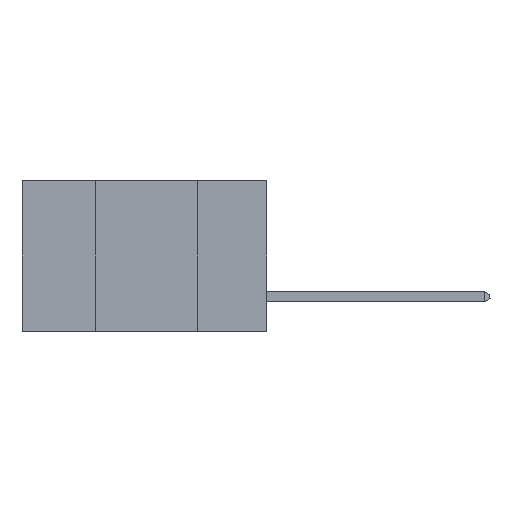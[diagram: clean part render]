
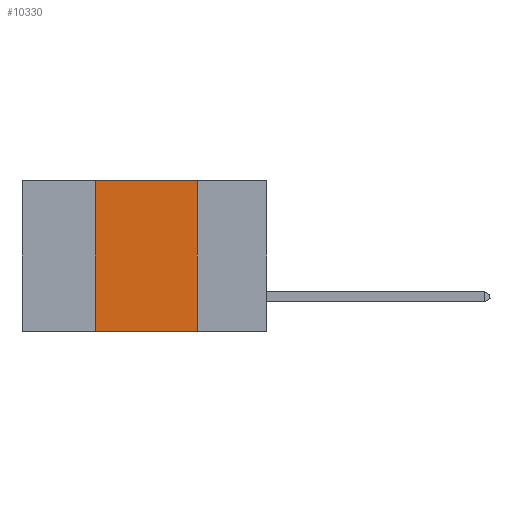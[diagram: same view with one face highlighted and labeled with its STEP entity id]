
A CAD part, left-side view. The second image highlights one B-rep face of the part: STEP entity #10330.
In plain terms, the highlighted planar face has unit normal (-1, 0, 0).
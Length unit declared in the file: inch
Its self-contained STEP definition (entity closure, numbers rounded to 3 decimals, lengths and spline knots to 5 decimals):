
#136 = CARTESIAN_POINT ( 'NONE',  ( 0., 0.42, 0. ) ) ;
#565 = ORIENTED_EDGE ( 'NONE', *, *, #669, .T. ) ;
#669 = EDGE_CURVE ( 'NONE', #7024, #15433, #6552, .T. ) ;
#1133 = VECTOR ( 'NONE', #11298, 39.37008 ) ;
#1370 = CARTESIAN_POINT ( 'NONE',  ( 0., 0.17, 0. ) ) ;
#1787 = EDGE_CURVE ( 'NONE', #2310, #15433, #2604, .T. ) ;
#2267 = LINE ( 'NONE', #8449, #11714 ) ;
#2310 = VERTEX_POINT ( 'NONE', #8445 ) ;
#2604 = LINE ( 'NONE', #1370, #10193 ) ;
#3486 = CARTESIAN_POINT ( 'NONE',  ( 0., 0.42, 0. ) ) ;
#3508 = ORIENTED_EDGE ( 'NONE', *, *, #1787, .F. ) ;
#3883 = DIRECTION ( 'NONE',  ( 0., 0., -1. ) ) ;
#5156 = DIRECTION ( 'NONE',  ( 0., -1., 0. ) ) ;
#6219 = EDGE_LOOP ( 'NONE', ( #3508, #15270, #9956, #565 ) ) ;
#6552 = LINE ( 'NONE', #9012, #15689 ) ;
#6774 = PLANE ( 'NONE',  #9988 ) ;
#7024 = VERTEX_POINT ( 'NONE', #11356 ) ;
#7658 = EDGE_CURVE ( 'NONE', #8710, #2310, #2267, .T. ) ;
#8445 = CARTESIAN_POINT ( 'NONE',  ( 0., 0.17, 0. ) ) ;
#8449 = CARTESIAN_POINT ( 'NONE',  ( 0., 0.6, 0. ) ) ;
#8710 = VERTEX_POINT ( 'NONE', #3486 ) ;
#9012 = CARTESIAN_POINT ( 'NONE',  ( 0., 0.6, -0.37 ) ) ;
#9956 = ORIENTED_EDGE ( 'NONE', *, *, #14484, .F. ) ;
#9988 = AXIS2_PLACEMENT_3D ( 'NONE', #14922, #13843, #3883 ) ;
#10193 = VECTOR ( 'NONE', #10383, 39.37008 ) ;
#10330 = ADVANCED_FACE ( 'NONE', ( #10565 ), #6774, .F. ) ;
#10383 = DIRECTION ( 'NONE',  ( 0., 0., -1. ) ) ;
#10565 = FACE_OUTER_BOUND ( 'NONE', #6219, .T. ) ;
#11298 = DIRECTION ( 'NONE',  ( 0., 0., 1. ) ) ;
#11356 = CARTESIAN_POINT ( 'NONE',  ( 0., 0.42, -0.37 ) ) ;
#11714 = VECTOR ( 'NONE', #13796, 39.37008 ) ;
#12895 = CARTESIAN_POINT ( 'NONE',  ( 0., 0.17, -0.37 ) ) ;
#13796 = DIRECTION ( 'NONE',  ( 0., -1., 0. ) ) ;
#13818 = LINE ( 'NONE', #136, #1133 ) ;
#13843 = DIRECTION ( 'NONE',  ( 1., 0., 0. ) ) ;
#14484 = EDGE_CURVE ( 'NONE', #7024, #8710, #13818, .T. ) ;
#14922 = CARTESIAN_POINT ( 'NONE',  ( 0., 0.6, 0. ) ) ;
#15270 = ORIENTED_EDGE ( 'NONE', *, *, #7658, .F. ) ;
#15433 = VERTEX_POINT ( 'NONE', #12895 ) ;
#15689 = VECTOR ( 'NONE', #5156, 39.37008 ) ;
